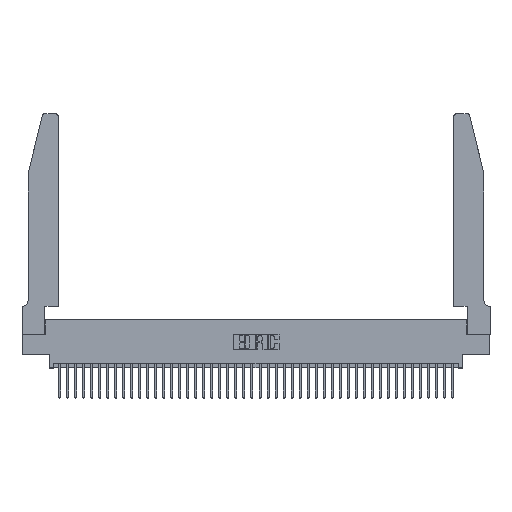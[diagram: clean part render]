
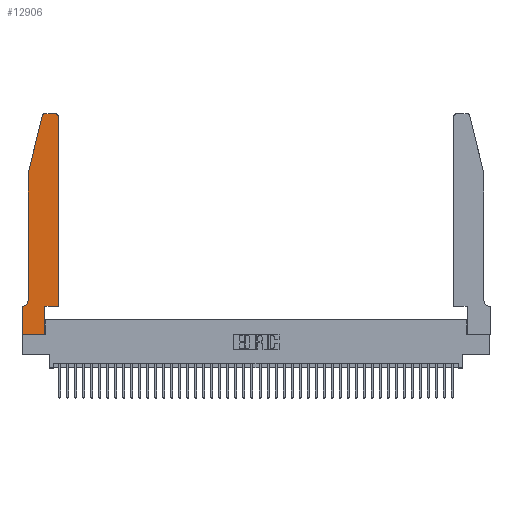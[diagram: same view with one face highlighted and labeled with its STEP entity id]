
A CAD part, top view. The second image highlights one B-rep face of the part: STEP entity #12906.
In plain terms, the highlighted planar face has unit normal (0, 0, 1).
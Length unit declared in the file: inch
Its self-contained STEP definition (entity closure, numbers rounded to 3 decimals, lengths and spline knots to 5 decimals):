
#226 = CARTESIAN_POINT ( 'NONE',  ( 0.0055, 0.35, 0.37 ) ) ;
#873 = DIRECTION ( 'NONE',  ( 0., 0., 1. ) ) ;
#1133 = EDGE_CURVE ( 'NONE', #28370, #39765, #40086, .T. ) ;
#2574 = CARTESIAN_POINT ( 'NONE',  ( 0.25487, 2.72718, 0.37 ) ) ;
#3221 = LINE ( 'NONE', #31916, #28765 ) ;
#3361 = ORIENTED_EDGE ( 'NONE', *, *, #1133, .T. ) ;
#3978 = DIRECTION ( 'NONE',  ( 0., 0., 1. ) ) ;
#4134 = VERTEX_POINT ( 'NONE', #14952 ) ;
#4889 = ORIENTED_EDGE ( 'NONE', *, *, #18825, .T. ) ;
#5791 = VECTOR ( 'NONE', #31168, 39.37008 ) ;
#6580 = DIRECTION ( 'NONE',  ( 0., 1., 0. ) ) ;
#8089 = CARTESIAN_POINT ( 'NONE',  ( 0.4205, 2.75, 0.37 ) ) ;
#8401 = CARTESIAN_POINT ( 'NONE',  ( 0., 0., 0.37 ) ) ;
#8530 = AXIS2_PLACEMENT_3D ( 'NONE', #38995, #19178, #42315 ) ;
#8614 = VERTEX_POINT ( 'NONE', #26882 ) ;
#8865 = CIRCLE ( 'NONE', #20864, 0.03 ) ;
#9159 = ORIENTED_EDGE ( 'NONE', *, *, #15677, .T. ) ;
#9571 = EDGE_CURVE ( 'NONE', #39765, #27269, #17069, .T. ) ;
#10571 = EDGE_CURVE ( 'NONE', #11428, #31018, #38220, .T. ) ;
#11179 = VECTOR ( 'NONE', #34909, 39.37008 ) ;
#11428 = VERTEX_POINT ( 'NONE', #37818 ) ;
#11641 = LINE ( 'NONE', #23203, #19445 ) ;
#11741 = CARTESIAN_POINT ( 'NONE',  ( 0.4505, 0.35, 0.37 ) ) ;
#11860 = LINE ( 'NONE', #13549, #19674 ) ;
#12297 = ORIENTED_EDGE ( 'NONE', *, *, #32541, .T. ) ;
#12481 = PLANE ( 'NONE',  #8530 ) ;
#12906 = ADVANCED_FACE ( 'NONE', ( #32133 ), #12481, .T. ) ;
#13549 = CARTESIAN_POINT ( 'NONE',  ( 0.0755, 0.35, 0.37 ) ) ;
#14620 = EDGE_CURVE ( 'NONE', #29209, #11428, #27396, .T. ) ;
#14952 = CARTESIAN_POINT ( 'NONE',  ( 0., 0., 0.37 ) ) ;
#15256 = VECTOR ( 'NONE', #35091, 39.37008 ) ;
#15677 = EDGE_CURVE ( 'NONE', #38770, #8614, #11641, .T. ) ;
#16773 = DIRECTION ( 'NONE',  ( 0., 0., -1. ) ) ;
#17069 = LINE ( 'NONE', #22015, #42445 ) ;
#17398 = CARTESIAN_POINT ( 'NONE',  ( 0., 0.35, 0.37 ) ) ;
#17642 = VERTEX_POINT ( 'NONE', #226 ) ;
#18374 = EDGE_CURVE ( 'NONE', #17642, #21296, #11860, .T. ) ;
#18825 = EDGE_CURVE ( 'NONE', #4134, #38770, #38266, .T. ) ;
#19178 = DIRECTION ( 'NONE',  ( 0., 0., 1. ) ) ;
#19445 = VECTOR ( 'NONE', #6580, 39.37008 ) ;
#19664 = EDGE_CURVE ( 'NONE', #27269, #17642, #24768, .T. ) ;
#19674 = VECTOR ( 'NONE', #33403, 39.37008 ) ;
#19716 = ORIENTED_EDGE ( 'NONE', *, *, #18374, .T. ) ;
#20487 = CARTESIAN_POINT ( 'NONE',  ( 0.0755, 2., 0.37 ) ) ;
#20830 = EDGE_CURVE ( 'NONE', #21296, #4134, #24151, .T. ) ;
#20864 = AXIS2_PLACEMENT_3D ( 'NONE', #23957, #3978, #27291 ) ;
#20932 = CARTESIAN_POINT ( 'NONE',  ( 0.4205, 2.72, 0.37 ) ) ;
#21296 = VERTEX_POINT ( 'NONE', #17398 ) ;
#22015 = CARTESIAN_POINT ( 'NONE',  ( 0.0755, 2., 0.37 ) ) ;
#22112 = CARTESIAN_POINT ( 'NONE',  ( 0., 0., 0.37 ) ) ;
#22788 = ORIENTED_EDGE ( 'NONE', *, *, #10571, .T. ) ;
#23203 = CARTESIAN_POINT ( 'NONE',  ( 0.2865, 0.35, 0.37 ) ) ;
#23299 = AXIS2_PLACEMENT_3D ( 'NONE', #20932, #873, #24269 ) ;
#23482 = ORIENTED_EDGE ( 'NONE', *, *, #20830, .T. ) ;
#23957 = CARTESIAN_POINT ( 'NONE',  ( 0.284, 2.72, 0.37 ) ) ;
#24151 = LINE ( 'NONE', #8401, #15256 ) ;
#24269 = DIRECTION ( 'NONE',  ( 1., 0., 0. ) ) ;
#24432 = CARTESIAN_POINT ( 'NONE',  ( 0.4505, 0.35, 0.37 ) ) ;
#24579 = DIRECTION ( 'NONE',  ( 0., 1., 0. ) ) ;
#24768 = CIRCLE ( 'NONE', #40881, 0.07 ) ;
#25282 = CARTESIAN_POINT ( 'NONE',  ( 0.4505, 0.35, 0.37 ) ) ;
#25793 = EDGE_CURVE ( 'NONE', #31018, #28851, #3221, .T. ) ;
#26882 = CARTESIAN_POINT ( 'NONE',  ( 0.2865, 0.35, 0.37 ) ) ;
#27056 = CARTESIAN_POINT ( 'NONE',  ( 0.0755, 0.42, 0.37 ) ) ;
#27269 = VERTEX_POINT ( 'NONE', #27056 ) ;
#27291 = DIRECTION ( 'NONE',  ( 1., 0., 0. ) ) ;
#27396 = LINE ( 'NONE', #24432, #35092 ) ;
#27884 = CARTESIAN_POINT ( 'NONE',  ( 0.0755, 2., 0.37 ) ) ;
#27956 = EDGE_CURVE ( 'NONE', #28851, #28370, #8865, .T. ) ;
#28370 = VERTEX_POINT ( 'NONE', #2574 ) ;
#28765 = VECTOR ( 'NONE', #41766, 39.37008 ) ;
#28771 = DIRECTION ( 'NONE',  ( 1., 0., 0. ) ) ;
#28851 = VERTEX_POINT ( 'NONE', #38590 ) ;
#29077 = ORIENTED_EDGE ( 'NONE', *, *, #19664, .T. ) ;
#29209 = VERTEX_POINT ( 'NONE', #25282 ) ;
#29421 = ORIENTED_EDGE ( 'NONE', *, *, #27956, .T. ) ;
#31018 = VERTEX_POINT ( 'NONE', #8089 ) ;
#31168 = DIRECTION ( 'NONE',  ( -0.239, -0.971, 0. ) ) ;
#31733 = ORIENTED_EDGE ( 'NONE', *, *, #14620, .T. ) ;
#31916 = CARTESIAN_POINT ( 'NONE',  ( 0.2605, 2.75, 0.37 ) ) ;
#32133 = FACE_OUTER_BOUND ( 'NONE', #36324, .T. ) ;
#32257 = CARTESIAN_POINT ( 'NONE',  ( 0.2865, 0., 0.37 ) ) ;
#32541 = EDGE_CURVE ( 'NONE', #8614, #29209, #36597, .T. ) ;
#33403 = DIRECTION ( 'NONE',  ( -1., 0., 0. ) ) ;
#34909 = DIRECTION ( 'NONE',  ( 1., 0., 0. ) ) ;
#35091 = DIRECTION ( 'NONE',  ( 0., -1., 0. ) ) ;
#35092 = VECTOR ( 'NONE', #24579, 39.37008 ) ;
#36324 = EDGE_LOOP ( 'NONE', ( #38273, #29421, #3361, #41668, #29077, #19716, #23482, #4889, #9159, #12297, #31733, #22788 ) ) ;
#36597 = LINE ( 'NONE', #11741, #11179 ) ;
#36634 = CARTESIAN_POINT ( 'NONE',  ( 0.0055, 0.42, 0.37 ) ) ;
#37258 = VECTOR ( 'NONE', #28771, 39.37008 ) ;
#37818 = CARTESIAN_POINT ( 'NONE',  ( 0.4505, 2.72, 0.37 ) ) ;
#38220 = CIRCLE ( 'NONE', #23299, 0.03 ) ;
#38266 = LINE ( 'NONE', #22112, #37258 ) ;
#38273 = ORIENTED_EDGE ( 'NONE', *, *, #25793, .T. ) ;
#38590 = CARTESIAN_POINT ( 'NONE',  ( 0.284, 2.75, 0.37 ) ) ;
#38770 = VERTEX_POINT ( 'NONE', #32257 ) ;
#38995 = CARTESIAN_POINT ( 'NONE',  ( 0., 0.35, 0.37 ) ) ;
#39765 = VERTEX_POINT ( 'NONE', #20487 ) ;
#39982 = DIRECTION ( 'NONE',  ( -1., 0., 0. ) ) ;
#40086 = LINE ( 'NONE', #27884, #5791 ) ;
#40881 = AXIS2_PLACEMENT_3D ( 'NONE', #36634, #16773, #39982 ) ;
#41668 = ORIENTED_EDGE ( 'NONE', *, *, #9571, .T. ) ;
#41766 = DIRECTION ( 'NONE',  ( -1., 0., 0. ) ) ;
#41800 = DIRECTION ( 'NONE',  ( 0., -1., 0. ) ) ;
#42315 = DIRECTION ( 'NONE',  ( 1., 0., 0. ) ) ;
#42445 = VECTOR ( 'NONE', #41800, 39.37008 ) ;
